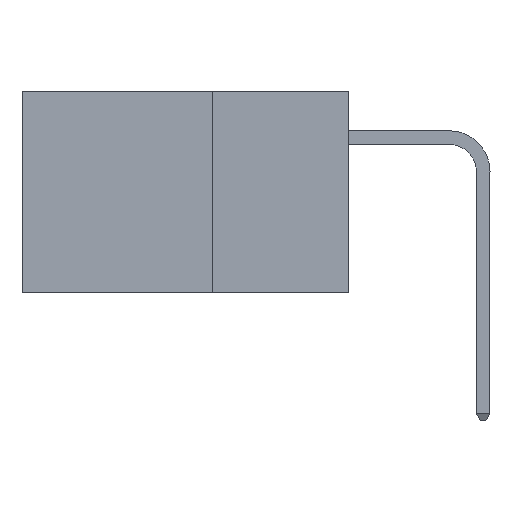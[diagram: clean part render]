
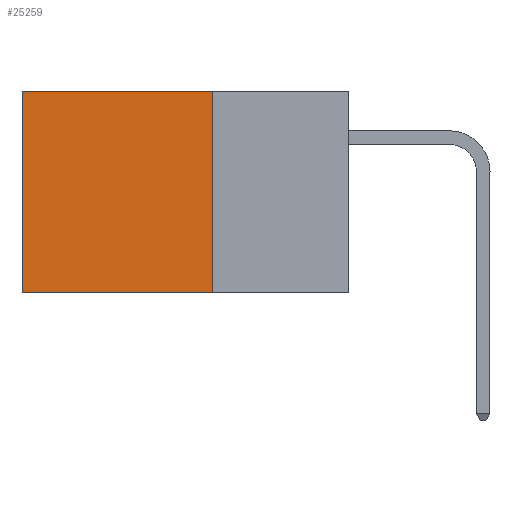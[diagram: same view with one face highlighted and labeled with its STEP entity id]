
A CAD part, left-side view. The second image highlights one B-rep face of the part: STEP entity #25259.
In plain terms, the highlighted planar face has unit normal (-1, 0, 0).
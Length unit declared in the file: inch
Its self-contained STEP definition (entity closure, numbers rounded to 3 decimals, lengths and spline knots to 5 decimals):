
#227 = LINE ( 'NONE', #28222, #28179 ) ;
#1533 = ORIENTED_EDGE ( 'NONE', *, *, #3229, .F. ) ;
#3100 = VECTOR ( 'NONE', #27994, 39.37008 ) ;
#3229 = EDGE_CURVE ( 'NONE', #20802, #17425, #6252, .T. ) ;
#3668 = FACE_OUTER_BOUND ( 'NONE', #23321, .T. ) ;
#3691 = LINE ( 'NONE', #10602, #12872 ) ;
#4763 = EDGE_CURVE ( 'NONE', #20802, #22613, #227, .T. ) ;
#6252 = LINE ( 'NONE', #24788, #16164 ) ;
#8249 = ORIENTED_EDGE ( 'NONE', *, *, #15451, .F. ) ;
#9930 = CARTESIAN_POINT ( 'NONE',  ( 0.2875, 0.6, 0. ) ) ;
#10602 = CARTESIAN_POINT ( 'NONE',  ( 0.2875, 0.25, -0.37 ) ) ;
#10943 = AXIS2_PLACEMENT_3D ( 'NONE', #28838, #28741, #19361 ) ;
#11197 = VERTEX_POINT ( 'NONE', #18107 ) ;
#12680 = EDGE_CURVE ( 'NONE', #22613, #11197, #15600, .T. ) ;
#12872 = VECTOR ( 'NONE', #26998, 39.37008 ) ;
#13115 = DIRECTION ( 'NONE',  ( 0., 0., -1. ) ) ;
#15451 = EDGE_CURVE ( 'NONE', #17425, #11197, #3691, .T. ) ;
#15600 = LINE ( 'NONE', #23464, #3100 ) ;
#16164 = VECTOR ( 'NONE', #13115, 39.37008 ) ;
#17132 = PLANE ( 'NONE',  #10943 ) ;
#17425 = VERTEX_POINT ( 'NONE', #18371 ) ;
#18107 = CARTESIAN_POINT ( 'NONE',  ( 0.2875, 0.6, -0.37 ) ) ;
#18371 = CARTESIAN_POINT ( 'NONE',  ( 0.2875, 0.25, -0.37 ) ) ;
#19257 = DIRECTION ( 'NONE',  ( 0., 1., 0. ) ) ;
#19361 = DIRECTION ( 'NONE',  ( 0., 0., -1. ) ) ;
#20167 = ORIENTED_EDGE ( 'NONE', *, *, #4763, .T. ) ;
#20802 = VERTEX_POINT ( 'NONE', #21948 ) ;
#21407 = ORIENTED_EDGE ( 'NONE', *, *, #12680, .T. ) ;
#21948 = CARTESIAN_POINT ( 'NONE',  ( 0.2875, 0.25, 0. ) ) ;
#22613 = VERTEX_POINT ( 'NONE', #9930 ) ;
#23321 = EDGE_LOOP ( 'NONE', ( #21407, #8249, #1533, #20167 ) ) ;
#23464 = CARTESIAN_POINT ( 'NONE',  ( 0.2875, 0.6, 0. ) ) ;
#24788 = CARTESIAN_POINT ( 'NONE',  ( 0.2875, 0.25, 0. ) ) ;
#25259 = ADVANCED_FACE ( 'NONE', ( #3668 ), #17132, .F. ) ;
#26998 = DIRECTION ( 'NONE',  ( 0., 1., 0. ) ) ;
#27994 = DIRECTION ( 'NONE',  ( 0., 0., -1. ) ) ;
#28179 = VECTOR ( 'NONE', #19257, 39.37008 ) ;
#28222 = CARTESIAN_POINT ( 'NONE',  ( 0.2875, 0.25, 0. ) ) ;
#28741 = DIRECTION ( 'NONE',  ( 1., 0., 0. ) ) ;
#28838 = CARTESIAN_POINT ( 'NONE',  ( 0.2875, 0.25, 0. ) ) ;
